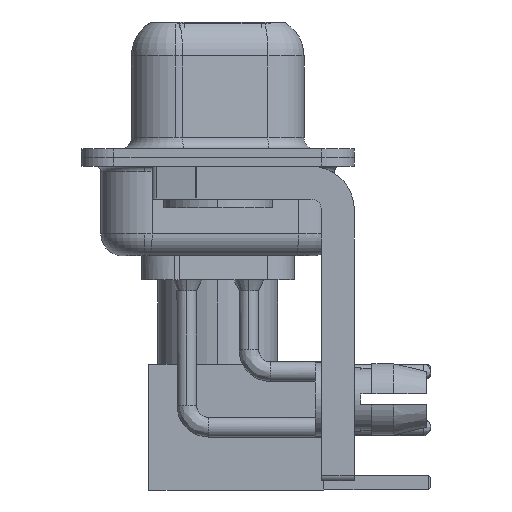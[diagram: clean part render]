
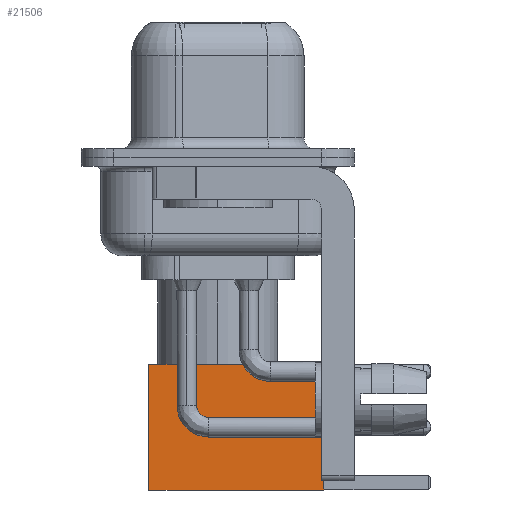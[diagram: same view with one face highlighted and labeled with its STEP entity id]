
A CAD part, left-side view. The second image highlights one B-rep face of the part: STEP entity #21506.
In plain terms, the highlighted face is planar.
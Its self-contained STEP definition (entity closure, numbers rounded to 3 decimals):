
#578 = CARTESIAN_POINT ( 'NONE',  ( -2.875, 2.875, 0. ) ) ;
#637 = EDGE_CURVE ( 'NONE', #24145, #10384, #10016, .T. ) ;
#1135 = CARTESIAN_POINT ( 'NONE',  ( -2.875, 2.875, 0. ) ) ;
#2090 = PLANE ( 'NONE',  #16647 ) ;
#3970 = ORIENTED_EDGE ( 'NONE', *, *, #12924, .F. ) ;
#4017 = VECTOR ( 'NONE', #4861, 1000. ) ;
#4104 = VECTOR ( 'NONE', #7071, 1000. ) ;
#4861 = DIRECTION ( 'NONE',  ( -1., 0., 0. ) ) ;
#5148 = LINE ( 'NONE', #20931, #16719 ) ;
#6052 = FACE_OUTER_BOUND ( 'NONE', #20372, .T. ) ;
#6201 = DIRECTION ( 'NONE',  ( 0., 0., 1. ) ) ;
#7071 = DIRECTION ( 'NONE',  ( 0., 0., -1. ) ) ;
#7597 = DIRECTION ( 'NONE',  ( -1., 0., 0. ) ) ;
#8607 = CARTESIAN_POINT ( 'NONE',  ( 0., 2.875, 0. ) ) ;
#9263 = DIRECTION ( 'NONE',  ( 0., 0., -1. ) ) ;
#10016 = LINE ( 'NONE', #13828, #13009 ) ;
#10384 = VERTEX_POINT ( 'NONE', #17726 ) ;
#11012 = EDGE_CURVE ( 'NONE', #12582, #13334, #18580, .T. ) ;
#11050 = ORIENTED_EDGE ( 'NONE', *, *, #16136, .T. ) ;
#12582 = VERTEX_POINT ( 'NONE', #23507 ) ;
#12883 = CARTESIAN_POINT ( 'NONE',  ( 2.875, 2.875, 8. ) ) ;
#12924 = EDGE_CURVE ( 'NONE', #10384, #13334, #24387, .T. ) ;
#13009 = VECTOR ( 'NONE', #7597, 1000. ) ;
#13334 = VERTEX_POINT ( 'NONE', #578 ) ;
#13828 = CARTESIAN_POINT ( 'NONE',  ( 0., 2.875, 8. ) ) ;
#16136 = EDGE_CURVE ( 'NONE', #24145, #12582, #5148, .T. ) ;
#16647 = AXIS2_PLACEMENT_3D ( 'NONE', #21716, #17723, #6201 ) ;
#16719 = VECTOR ( 'NONE', #9263, 1000. ) ;
#17723 = DIRECTION ( 'NONE',  ( 0., 1., 0. ) ) ;
#17726 = CARTESIAN_POINT ( 'NONE',  ( -2.875, 2.875, 8. ) ) ;
#18580 = LINE ( 'NONE', #8607, #4017 ) ;
#20372 = EDGE_LOOP ( 'NONE', ( #11050, #20566, #3970, #21941 ) ) ;
#20566 = ORIENTED_EDGE ( 'NONE', *, *, #11012, .T. ) ;
#20931 = CARTESIAN_POINT ( 'NONE',  ( 2.875, 2.875, 0. ) ) ;
#21506 = ADVANCED_FACE ( 'NONE', ( #6052 ), #2090, .T. ) ;
#21716 = CARTESIAN_POINT ( 'NONE',  ( 2.875, 2.875, 0. ) ) ;
#21941 = ORIENTED_EDGE ( 'NONE', *, *, #637, .F. ) ;
#23507 = CARTESIAN_POINT ( 'NONE',  ( 2.875, 2.875, 0. ) ) ;
#24145 = VERTEX_POINT ( 'NONE', #12883 ) ;
#24387 = LINE ( 'NONE', #1135, #4104 ) ;
